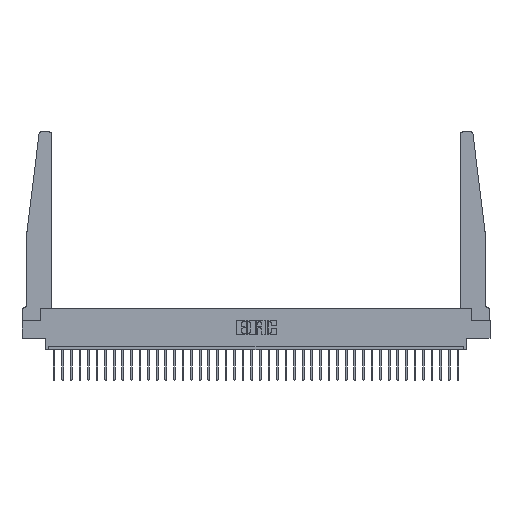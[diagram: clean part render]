
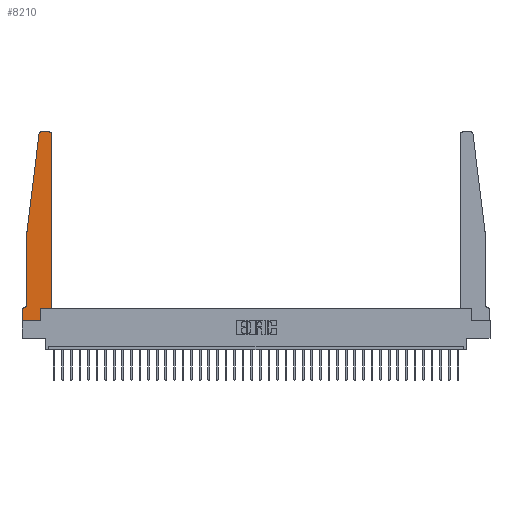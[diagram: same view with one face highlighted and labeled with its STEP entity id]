
A CAD part, top view. The second image highlights one B-rep face of the part: STEP entity #8210.
In plain terms, the highlighted planar face has unit normal (0, 0, 1).
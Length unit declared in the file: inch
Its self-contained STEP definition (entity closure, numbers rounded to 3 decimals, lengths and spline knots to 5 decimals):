
#264 = EDGE_CURVE ( 'NONE', #18639, #17428, #14941, .T. ) ;
#877 = CARTESIAN_POINT ( 'NONE',  ( 0.395, 2.75, 0.37 ) ) ;
#1128 = DIRECTION ( 'NONE',  ( 0., 0., 1. ) ) ;
#1145 = LINE ( 'NONE', #27727, #10563 ) ;
#1467 = CARTESIAN_POINT ( 'NONE',  ( 0.395, 2.72, 0.37 ) ) ;
#1519 = ORIENTED_EDGE ( 'NONE', *, *, #18584, .T. ) ;
#1686 = CARTESIAN_POINT ( 'NONE',  ( 0.065, 0.1875, 0.37 ) ) ;
#1694 = EDGE_CURVE ( 'NONE', #14795, #7151, #27535, .T. ) ;
#1760 = FACE_OUTER_BOUND ( 'NONE', #1825, .T. ) ;
#1825 = EDGE_LOOP ( 'NONE', ( #1519, #24940, #4288, #6720, #29340, #8894, #32974, #27129, #15515, #16245, #13848, #23138 ) ) ;
#1937 = VECTOR ( 'NONE', #21718, 39.37008 ) ;
#2091 = DIRECTION ( 'NONE',  ( 0., -1., 0. ) ) ;
#3132 = DIRECTION ( 'NONE',  ( 0., 1., 0. ) ) ;
#3805 = EDGE_CURVE ( 'NONE', #34177, #24078, #16850, .T. ) ;
#3917 = DIRECTION ( 'NONE',  ( 0., -1., 0. ) ) ;
#3992 = DIRECTION ( 'NONE',  ( 1., 0., 0. ) ) ;
#4288 = ORIENTED_EDGE ( 'NONE', *, *, #31180, .T. ) ;
#5096 = VECTOR ( 'NONE', #22777, 39.37008 ) ;
#5539 = LINE ( 'NONE', #26576, #1937 ) ;
#5944 = EDGE_CURVE ( 'NONE', #17428, #34177, #32322, .T. ) ;
#6370 = VERTEX_POINT ( 'NONE', #13696 ) ;
#6720 = ORIENTED_EDGE ( 'NONE', *, *, #8438, .T. ) ;
#7105 = CARTESIAN_POINT ( 'NONE',  ( 0.425, 0.18, 0.37 ) ) ;
#7151 = VERTEX_POINT ( 'NONE', #16527 ) ;
#7310 = CARTESIAN_POINT ( 'NONE',  ( 0.065, 1.25, 0.37 ) ) ;
#7503 = CARTESIAN_POINT ( 'NONE',  ( 0.065, 1.25, 0.37 ) ) ;
#7957 = CARTESIAN_POINT ( 'NONE',  ( 0., 0., 0.37 ) ) ;
#8210 = ADVANCED_FACE ( 'NONE', ( #1760 ), #17095, .T. ) ;
#8295 = CARTESIAN_POINT ( 'NONE',  ( 0.27653, 2.72, 0.37 ) ) ;
#8304 = CARTESIAN_POINT ( 'NONE',  ( 0.2605, 0.18, 0.37 ) ) ;
#8438 = EDGE_CURVE ( 'NONE', #10726, #6370, #12531, .T. ) ;
#8894 = ORIENTED_EDGE ( 'NONE', *, *, #10216, .T. ) ;
#9070 = CARTESIAN_POINT ( 'NONE',  ( 0., 0.1875, 0.37 ) ) ;
#9174 = DIRECTION ( 'NONE',  ( 0., 0., -1. ) ) ;
#9601 = LINE ( 'NONE', #7503, #29432 ) ;
#9664 = LINE ( 'NONE', #33815, #24543 ) ;
#10105 = DIRECTION ( 'NONE',  ( -0.122, -0.992, 0. ) ) ;
#10216 = EDGE_CURVE ( 'NONE', #21845, #28866, #20149, .T. ) ;
#10265 = CARTESIAN_POINT ( 'NONE',  ( 0., 0.1875, 0.37 ) ) ;
#10394 = EDGE_CURVE ( 'NONE', #6370, #21845, #32312, .T. ) ;
#10405 = CARTESIAN_POINT ( 'NONE',  ( 0.425, 0.18, 0.37 ) ) ;
#10563 = VECTOR ( 'NONE', #3917, 39.37008 ) ;
#10726 = VERTEX_POINT ( 'NONE', #17490 ) ;
#10785 = CARTESIAN_POINT ( 'NONE',  ( 0.425, 0.18, 0.37 ) ) ;
#11224 = AXIS2_PLACEMENT_3D ( 'NONE', #32980, #9174, #28961 ) ;
#11436 = DIRECTION ( 'NONE',  ( 1., 0., 0. ) ) ;
#12531 = LINE ( 'NONE', #7310, #12602 ) ;
#12602 = VECTOR ( 'NONE', #2091, 39.37008 ) ;
#13378 = AXIS2_PLACEMENT_3D ( 'NONE', #9070, #33229, #20046 ) ;
#13441 = CARTESIAN_POINT ( 'NONE',  ( 0.425, 2.72, 0.37 ) ) ;
#13596 = CARTESIAN_POINT ( 'NONE',  ( 0.015, 0.1875, 0.37 ) ) ;
#13696 = CARTESIAN_POINT ( 'NONE',  ( 0.065, 0.2375, 0.37 ) ) ;
#13848 = ORIENTED_EDGE ( 'NONE', *, *, #5944, .T. ) ;
#13887 = VECTOR ( 'NONE', #3992, 39.37008 ) ;
#14795 = VERTEX_POINT ( 'NONE', #27284 ) ;
#14941 = LINE ( 'NONE', #7105, #13887 ) ;
#15076 = EDGE_CURVE ( 'NONE', #24281, #19015, #30406, .T. ) ;
#15515 = ORIENTED_EDGE ( 'NONE', *, *, #32521, .T. ) ;
#16245 = ORIENTED_EDGE ( 'NONE', *, *, #264, .T. ) ;
#16413 = AXIS2_PLACEMENT_3D ( 'NONE', #8295, #24485, #11436 ) ;
#16527 = CARTESIAN_POINT ( 'NONE',  ( 0.24675, 2.72367, 0.37 ) ) ;
#16780 = VECTOR ( 'NONE', #3132, 39.37008 ) ;
#16850 = CIRCLE ( 'NONE', #34007, 0.03 ) ;
#17095 = PLANE ( 'NONE',  #13378 ) ;
#17428 = VERTEX_POINT ( 'NONE', #10405 ) ;
#17490 = CARTESIAN_POINT ( 'NONE',  ( 0.065, 1.25, 0.37 ) ) ;
#18584 = EDGE_CURVE ( 'NONE', #24078, #14795, #5539, .T. ) ;
#18639 = VERTEX_POINT ( 'NONE', #8304 ) ;
#19015 = VERTEX_POINT ( 'NONE', #34176 ) ;
#20011 = CARTESIAN_POINT ( 'NONE',  ( 0., 0., 0.37 ) ) ;
#20046 = DIRECTION ( 'NONE',  ( 1., 0., 0. ) ) ;
#20149 = LINE ( 'NONE', #1686, #22329 ) ;
#20309 = DIRECTION ( 'NONE',  ( 0., 1., 0. ) ) ;
#21718 = DIRECTION ( 'NONE',  ( -1., 0., 0. ) ) ;
#21845 = VERTEX_POINT ( 'NONE', #13596 ) ;
#22329 = VECTOR ( 'NONE', #27939, 39.37008 ) ;
#22777 = DIRECTION ( 'NONE',  ( 1., 0., 0. ) ) ;
#23138 = ORIENTED_EDGE ( 'NONE', *, *, #3805, .T. ) ;
#24078 = VERTEX_POINT ( 'NONE', #877 ) ;
#24281 = VERTEX_POINT ( 'NONE', #7957 ) ;
#24485 = DIRECTION ( 'NONE',  ( 0., 0., 1. ) ) ;
#24543 = VECTOR ( 'NONE', #20309, 39.37008 ) ;
#24940 = ORIENTED_EDGE ( 'NONE', *, *, #1694, .T. ) ;
#26576 = CARTESIAN_POINT ( 'NONE',  ( 0.25, 2.75, 0.37 ) ) ;
#27129 = ORIENTED_EDGE ( 'NONE', *, *, #15076, .T. ) ;
#27284 = CARTESIAN_POINT ( 'NONE',  ( 0.27653, 2.75, 0.37 ) ) ;
#27535 = CIRCLE ( 'NONE', #16413, 0.03 ) ;
#27727 = CARTESIAN_POINT ( 'NONE',  ( 0., 0., 0.37 ) ) ;
#27939 = DIRECTION ( 'NONE',  ( -1., 0., 0. ) ) ;
#28866 = VERTEX_POINT ( 'NONE', #10265 ) ;
#28961 = DIRECTION ( 'NONE',  ( -1., 0., 0. ) ) ;
#29340 = ORIENTED_EDGE ( 'NONE', *, *, #10394, .T. ) ;
#29401 = EDGE_CURVE ( 'NONE', #28866, #24281, #1145, .T. ) ;
#29432 = VECTOR ( 'NONE', #10105, 39.37008 ) ;
#30406 = LINE ( 'NONE', #20011, #5096 ) ;
#30650 = DIRECTION ( 'NONE',  ( 1., 0., 0. ) ) ;
#31180 = EDGE_CURVE ( 'NONE', #7151, #10726, #9601, .T. ) ;
#32312 = CIRCLE ( 'NONE', #11224, 0.05 ) ;
#32322 = LINE ( 'NONE', #10785, #16780 ) ;
#32521 = EDGE_CURVE ( 'NONE', #19015, #18639, #9664, .T. ) ;
#32974 = ORIENTED_EDGE ( 'NONE', *, *, #29401, .T. ) ;
#32980 = CARTESIAN_POINT ( 'NONE',  ( 0.015, 0.2375, 0.37 ) ) ;
#33229 = DIRECTION ( 'NONE',  ( 0., 0., 1. ) ) ;
#33815 = CARTESIAN_POINT ( 'NONE',  ( 0.2605, 0.18, 0.37 ) ) ;
#34007 = AXIS2_PLACEMENT_3D ( 'NONE', #1467, #1128, #30650 ) ;
#34176 = CARTESIAN_POINT ( 'NONE',  ( 0.2605, 0., 0.37 ) ) ;
#34177 = VERTEX_POINT ( 'NONE', #13441 ) ;
